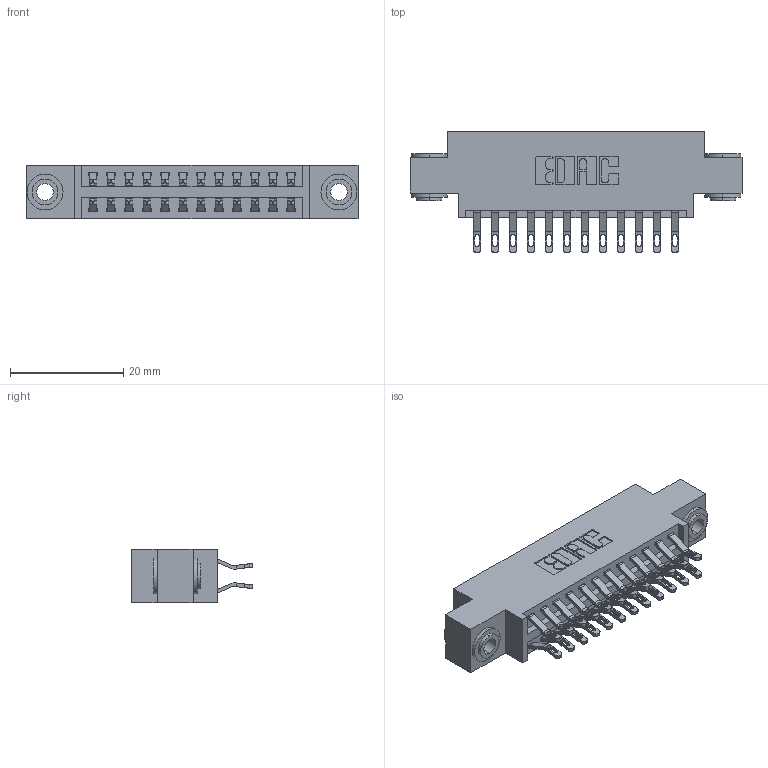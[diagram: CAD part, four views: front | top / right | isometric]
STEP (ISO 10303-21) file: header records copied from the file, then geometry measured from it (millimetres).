
FILE_DESCRIPTION (( 'STEP AP203' ), '1' );
FILE_NAME ('346-024-555-803.STEP', '2022-05-18T23:56:29', ( '' ), ( '' ), 'SwSTEP 2.0', 'SolidWorks 2020', '' );
FILE_SCHEMA (( 'CONFIG_CONTROL_DESIGN' ));
Length unit declared in the file: inch
Products named in the file (4): 346-024-555-803; 345-250-002_345-250-002-102; 346 Part_0.170 Offset - 0.156 Dia-TH; 345-292-001_555 Tail
Assembly tree (27 placements, depth 2):
  346-024-555-803
    346 Part_0.170 Offset - 0.156 Dia-TH
    345-292-001_555 Tail  x24
    345-250-002_345-250-002-102  x2
Bounding box: 58.67 x 21.46 x 9.4 mm (x, y, z)
Volume: 5404.7 mm3; surface area: 7634.1 mm2
Topology: 27 solids, 27 shells, 1570 faces, 4845 edges, 3226 vertices
Faces by surface type: plane 896, cylinder 666, cone 8
Entity records: 13394 total; most frequent: CARTESIAN_POINT 2267, ORIENTED_EDGE 2162, DIRECTION 2047, EDGE_CURVE 1081, VECTOR 857, LINE 857, VERTEX_POINT 718, AXIS2_PLACEMENT_3D 595
